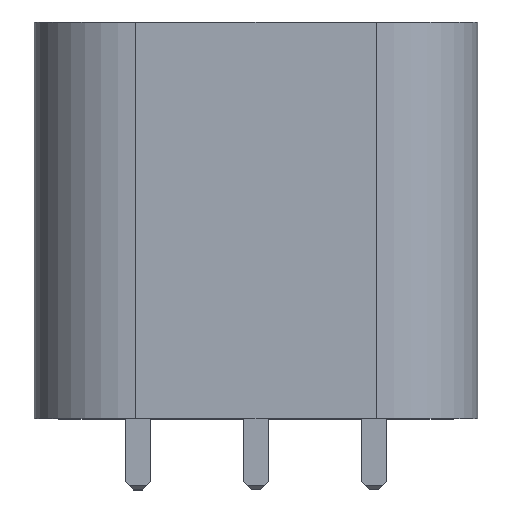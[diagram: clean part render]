
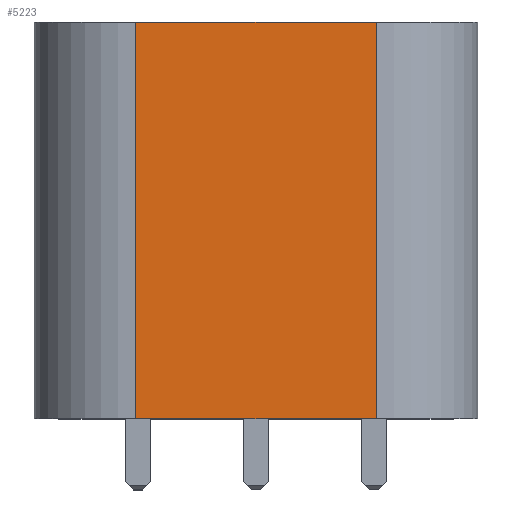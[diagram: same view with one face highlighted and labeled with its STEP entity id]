
A CAD part, top view. The second image highlights one B-rep face of the part: STEP entity #5223.
In plain terms, the highlighted planar face has unit normal (0, 0, 1).
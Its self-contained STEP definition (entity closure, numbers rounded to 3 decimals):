
#149 = EDGE_LOOP ( 'NONE', ( #3640, #3857, #1874, #587 ) ) ;
#228 = VECTOR ( 'NONE', #1528, 1000. ) ;
#263 = DIRECTION ( 'NONE',  ( 1., 0., 0. ) ) ;
#587 = ORIENTED_EDGE ( 'NONE', *, *, #3960, .T. ) ;
#1392 = VERTEX_POINT ( 'NONE', #1735 ) ;
#1414 = AXIS2_PLACEMENT_3D ( 'NONE', #6055, #3092, #4715 ) ;
#1452 = LINE ( 'NONE', #6110, #3077 ) ;
#1528 = DIRECTION ( 'NONE',  ( 0., -1., 0. ) ) ;
#1587 = CARTESIAN_POINT ( 'NONE',  ( 5.9, 19.5, 0. ) ) ;
#1735 = CARTESIAN_POINT ( 'NONE',  ( -5.9, 19.5, 0. ) ) ;
#1744 = PLANE ( 'NONE',  #1414 ) ;
#1874 = ORIENTED_EDGE ( 'NONE', *, *, #4753, .F. ) ;
#2024 = CARTESIAN_POINT ( 'NONE',  ( -5.9, 19.5, 0. ) ) ;
#2356 = DIRECTION ( 'NONE',  ( 1., 0., 0. ) ) ;
#2449 = VERTEX_POINT ( 'NONE', #4882 ) ;
#2568 = VECTOR ( 'NONE', #263, 1000. ) ;
#2575 = VECTOR ( 'NONE', #2356, 1000. ) ;
#2794 = CARTESIAN_POINT ( 'NONE',  ( -5.9, 0., 0. ) ) ;
#3017 = EDGE_CURVE ( 'NONE', #4536, #2449, #1452, .T. ) ;
#3042 = EDGE_CURVE ( 'NONE', #5331, #2449, #3299, .T. ) ;
#3077 = VECTOR ( 'NONE', #3728, 1000. ) ;
#3092 = DIRECTION ( 'NONE',  ( 0., 0., -1. ) ) ;
#3299 = LINE ( 'NONE', #2794, #2575 ) ;
#3568 = CARTESIAN_POINT ( 'NONE',  ( -5.9, 19.5, 0. ) ) ;
#3640 = ORIENTED_EDGE ( 'NONE', *, *, #3042, .T. ) ;
#3728 = DIRECTION ( 'NONE',  ( 0., -1., 0. ) ) ;
#3857 = ORIENTED_EDGE ( 'NONE', *, *, #3017, .F. ) ;
#3960 = EDGE_CURVE ( 'NONE', #1392, #5331, #4294, .T. ) ;
#4110 = FACE_OUTER_BOUND ( 'NONE', #149, .T. ) ;
#4294 = LINE ( 'NONE', #2024, #228 ) ;
#4536 = VERTEX_POINT ( 'NONE', #1587 ) ;
#4715 = DIRECTION ( 'NONE',  ( -1., 0., 0. ) ) ;
#4753 = EDGE_CURVE ( 'NONE', #1392, #4536, #4952, .T. ) ;
#4882 = CARTESIAN_POINT ( 'NONE',  ( 5.9, 0., 0. ) ) ;
#4952 = LINE ( 'NONE', #3568, #2568 ) ;
#5178 = CARTESIAN_POINT ( 'NONE',  ( -5.9, 0., 0. ) ) ;
#5223 = ADVANCED_FACE ( 'NONE', ( #4110 ), #1744, .F. ) ;
#5331 = VERTEX_POINT ( 'NONE', #5178 ) ;
#6055 = CARTESIAN_POINT ( 'NONE',  ( -5.9, 19.5, 0. ) ) ;
#6110 = CARTESIAN_POINT ( 'NONE',  ( 5.9, 19.5, 0. ) ) ;
